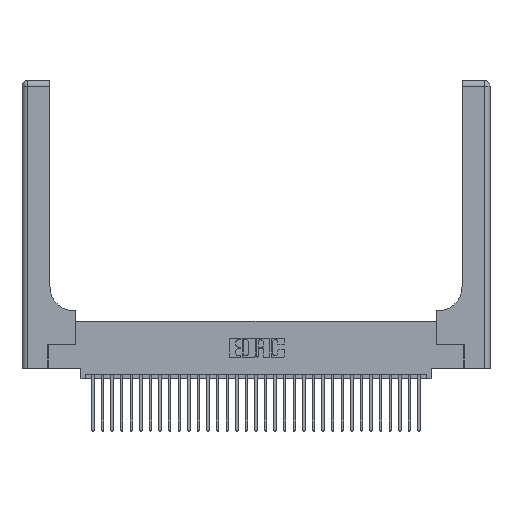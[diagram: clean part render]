
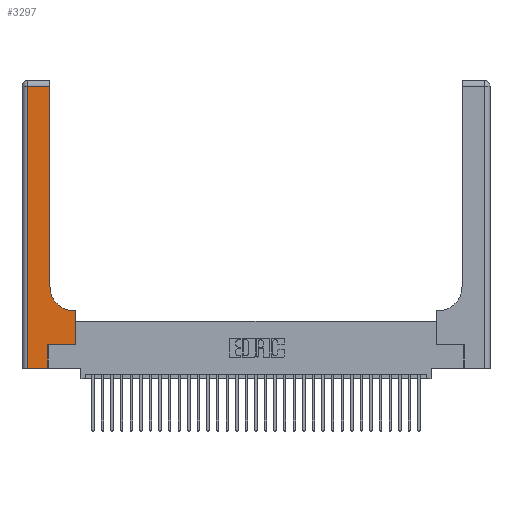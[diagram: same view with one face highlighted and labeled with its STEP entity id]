
A CAD part, top view. The second image highlights one B-rep face of the part: STEP entity #3297.
In plain terms, the highlighted planar face has unit normal (0, 0, 1).
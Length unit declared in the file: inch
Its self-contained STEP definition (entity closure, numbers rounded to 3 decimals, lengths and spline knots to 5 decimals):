
#695 = AXIS2_PLACEMENT_3D ( 'NONE', #12188, #20035, #9672 ) ;
#1533 = DIRECTION ( 'NONE',  ( 0., 1., 0. ) ) ;
#1685 = ORIENTED_EDGE ( 'NONE', *, *, #2633, .T. ) ;
#1791 = CARTESIAN_POINT ( 'NONE',  ( 0.06, 0., 0.37 ) ) ;
#2007 = VECTOR ( 'NONE', #6602, 39.37008 ) ;
#2161 = VECTOR ( 'NONE', #5629, 39.37008 ) ;
#2248 = ORIENTED_EDGE ( 'NONE', *, *, #6750, .T. ) ;
#2633 = EDGE_CURVE ( 'NONE', #13290, #2945, #32911, .T. ) ;
#2793 = CARTESIAN_POINT ( 'NONE',  ( 0.5415, 0.85, 0.37 ) ) ;
#2945 = VERTEX_POINT ( 'NONE', #30357 ) ;
#3110 = DIRECTION ( 'NONE',  ( -1., 0., 0. ) ) ;
#3297 = ADVANCED_FACE ( 'NONE', ( #7581 ), #4565, .F. ) ;
#3330 = ORIENTED_EDGE ( 'NONE', *, *, #24009, .T. ) ;
#3432 = VECTOR ( 'NONE', #16385, 39.37008 ) ;
#4565 = PLANE ( 'NONE',  #695 ) ;
#4684 = DIRECTION ( 'NONE',  ( 1., 0., 0. ) ) ;
#5629 = DIRECTION ( 'NONE',  ( 1., 0., 0. ) ) ;
#5922 = ORIENTED_EDGE ( 'NONE', *, *, #25870, .T. ) ;
#6152 = CARTESIAN_POINT ( 'NONE',  ( 0.5585, 0.25, 0.37 ) ) ;
#6602 = DIRECTION ( 'NONE',  ( -1., 0., 0. ) ) ;
#6750 = EDGE_CURVE ( 'NONE', #32011, #29470, #17994, .T. ) ;
#7321 = CARTESIAN_POINT ( 'NONE',  ( 0.06, 2.94, 0.37 ) ) ;
#7351 = ORIENTED_EDGE ( 'NONE', *, *, #9637, .T. ) ;
#7581 = FACE_OUTER_BOUND ( 'NONE', #12810, .T. ) ;
#8231 = ORIENTED_EDGE ( 'NONE', *, *, #30353, .T. ) ;
#8926 = AXIS2_PLACEMENT_3D ( 'NONE', #2793, #13174, #31376 ) ;
#8937 = LINE ( 'NONE', #12088, #2007 ) ;
#9300 = CARTESIAN_POINT ( 'NONE',  ( 0.5585, 0.6, 0.37 ) ) ;
#9637 = EDGE_CURVE ( 'NONE', #25580, #24775, #8937, .T. ) ;
#9672 = DIRECTION ( 'NONE',  ( -1., 0., 0. ) ) ;
#11870 = LINE ( 'NONE', #13499, #18406 ) ;
#12088 = CARTESIAN_POINT ( 'NONE',  ( 0.2915, 0.6, 0.37 ) ) ;
#12188 = CARTESIAN_POINT ( 'NONE',  ( 0., 3., 0.37 ) ) ;
#12810 = EDGE_LOOP ( 'NONE', ( #2248, #3330, #27782, #1685, #23430, #8231, #15566, #7351, #5922 ) ) ;
#13174 = DIRECTION ( 'NONE',  ( 0., 0., -1. ) ) ;
#13237 = CARTESIAN_POINT ( 'NONE',  ( 0.5585, 0.25, 0.37 ) ) ;
#13290 = VERTEX_POINT ( 'NONE', #1791 ) ;
#13401 = LINE ( 'NONE', #24462, #32538 ) ;
#13499 = CARTESIAN_POINT ( 'NONE',  ( 0., 2.94, 0.37 ) ) ;
#14056 = VERTEX_POINT ( 'NONE', #7321 ) ;
#15072 = VECTOR ( 'NONE', #17893, 39.37008 ) ;
#15566 = ORIENTED_EDGE ( 'NONE', *, *, #33323, .T. ) ;
#16234 = CARTESIAN_POINT ( 'NONE',  ( 0.269, 0.25, 0.37 ) ) ;
#16385 = DIRECTION ( 'NONE',  ( 0., -1., 0. ) ) ;
#17782 = EDGE_CURVE ( 'NONE', #2945, #26686, #13401, .T. ) ;
#17893 = DIRECTION ( 'NONE',  ( 0., 1., 0. ) ) ;
#17994 = LINE ( 'NONE', #33092, #26968 ) ;
#18406 = VECTOR ( 'NONE', #3110, 39.37008 ) ;
#19146 = CARTESIAN_POINT ( 'NONE',  ( 0.5415, 0.6, 0.37 ) ) ;
#19243 = VERTEX_POINT ( 'NONE', #6152 ) ;
#19318 = CARTESIAN_POINT ( 'NONE',  ( 0.06, 3., 0.37 ) ) ;
#20035 = DIRECTION ( 'NONE',  ( 0., 0., -1. ) ) ;
#20255 = CARTESIAN_POINT ( 'NONE',  ( 0.2915, 0.85, 0.37 ) ) ;
#20484 = CARTESIAN_POINT ( 'NONE',  ( 0.2915, 2.94, 0.37 ) ) ;
#21745 = CARTESIAN_POINT ( 'NONE',  ( 0.269, 0.25, 0.37 ) ) ;
#22094 = LINE ( 'NONE', #16234, #2161 ) ;
#23430 = ORIENTED_EDGE ( 'NONE', *, *, #17782, .T. ) ;
#24009 = EDGE_CURVE ( 'NONE', #29470, #14056, #11870, .T. ) ;
#24316 = VECTOR ( 'NONE', #4684, 39.37008 ) ;
#24348 = CIRCLE ( 'NONE', #8926, 0.25 ) ;
#24462 = CARTESIAN_POINT ( 'NONE',  ( 0.269, 0., 0.37 ) ) ;
#24775 = VERTEX_POINT ( 'NONE', #19146 ) ;
#25580 = VERTEX_POINT ( 'NONE', #9300 ) ;
#25870 = EDGE_CURVE ( 'NONE', #24775, #32011, #24348, .T. ) ;
#26686 = VERTEX_POINT ( 'NONE', #21745 ) ;
#26968 = VECTOR ( 'NONE', #1533, 39.37008 ) ;
#26991 = CARTESIAN_POINT ( 'NONE',  ( 0., 0., 0.37 ) ) ;
#27782 = ORIENTED_EDGE ( 'NONE', *, *, #29793, .T. ) ;
#27863 = LINE ( 'NONE', #19318, #3432 ) ;
#28879 = LINE ( 'NONE', #13237, #15072 ) ;
#29470 = VERTEX_POINT ( 'NONE', #20484 ) ;
#29793 = EDGE_CURVE ( 'NONE', #14056, #13290, #27863, .T. ) ;
#30313 = DIRECTION ( 'NONE',  ( 0., 1., 0. ) ) ;
#30353 = EDGE_CURVE ( 'NONE', #26686, #19243, #22094, .T. ) ;
#30357 = CARTESIAN_POINT ( 'NONE',  ( 0.269, 0., 0.37 ) ) ;
#31376 = DIRECTION ( 'NONE',  ( 1., 0., 0. ) ) ;
#32011 = VERTEX_POINT ( 'NONE', #20255 ) ;
#32538 = VECTOR ( 'NONE', #30313, 39.37008 ) ;
#32911 = LINE ( 'NONE', #26991, #24316 ) ;
#33092 = CARTESIAN_POINT ( 'NONE',  ( 0.2915, 3., 0.37 ) ) ;
#33323 = EDGE_CURVE ( 'NONE', #19243, #25580, #28879, .T. ) ;
